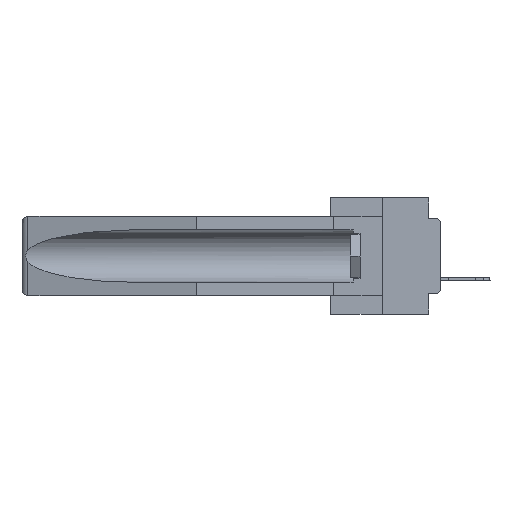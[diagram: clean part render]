
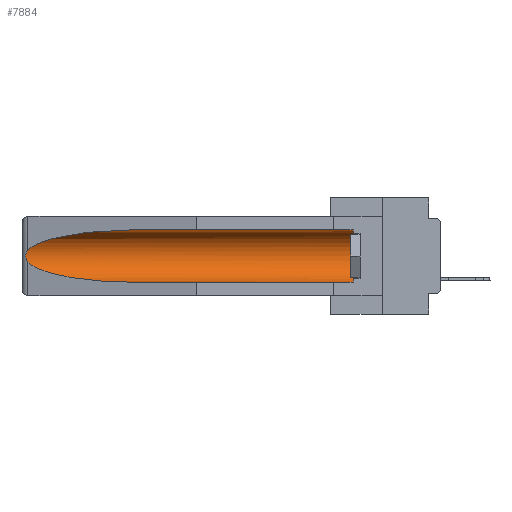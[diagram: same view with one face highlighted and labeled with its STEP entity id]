
A CAD part, left-side view. The second image highlights one B-rep face of the part: STEP entity #7884.
In plain terms, the highlighted cylindrical face has radius 2.857 mm (diameter 5.715 mm), a partial arc.
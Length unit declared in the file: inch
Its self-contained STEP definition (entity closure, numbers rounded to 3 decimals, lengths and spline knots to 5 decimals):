
#399 = CARTESIAN_POINT ( 'NONE',  ( 0.26537, 1.52718, -0.14972 ) ) ;
#456 = VECTOR ( 'NONE', #26872, 39.37008 ) ;
#866 = CARTESIAN_POINT ( 'NONE',  ( 0.155, -0.30754, -0.284 ) ) ;
#1058 = LINE ( 'NONE', #33928, #4656 ) ;
#1712 = VERTEX_POINT ( 'NONE', #8143 ) ;
#2428 = CARTESIAN_POINT ( 'NONE',  ( 0.155, 1.07973, -0.284 ) ) ;
#3092 = AXIS2_PLACEMENT_3D ( 'NONE', #14240, #19662, #25760 ) ;
#3195 = ORIENTED_EDGE ( 'NONE', *, *, #32228, .T. ) ;
#4011 = CARTESIAN_POINT ( 'NONE',  ( 0.25451, 1.48313, -0.09465 ) ) ;
#4656 = VECTOR ( 'NONE', #8696, 39.37008 ) ;
#5675 = CARTESIAN_POINT ( 'NONE',  ( 0.26537, 1.52718, -0.19328 ) ) ;
#5795 = CARTESIAN_POINT ( 'NONE',  ( 0.2673, 1.53269, -0.17917 ) ) ;
#6027 =( BOUNDED_CURVE ( )  B_SPLINE_CURVE ( 3, ( #21698, #19061, #21959, #36262 ),
 .UNSPECIFIED., .F., .F. ) 
 B_SPLINE_CURVE_WITH_KNOTS ( ( 4, 4 ),
 ( 0.1948, 1.5708 ),
 .UNSPECIFIED. ) 
 CURVE ( )  GEOMETRIC_REPRESENTATION_ITEM ( )  RATIONAL_B_SPLINE_CURVE ( ( 1., 0.848, 0.848, 1. ) ) 
 REPRESENTATION_ITEM ( '' )  );
#6773 = EDGE_CURVE ( 'NONE', #31456, #27522, #19392, .T. ) ;
#7884 = ADVANCED_FACE ( 'NONE', ( #23333 ), #31777, .F. ) ;
#8102 = DIRECTION ( 'NONE',  ( 0., -1., 0. ) ) ;
#8143 = CARTESIAN_POINT ( 'NONE',  ( 0.26537, 1.52718, -0.14972 ) ) ;
#8635 = CARTESIAN_POINT ( 'NONE',  ( 0.26597, 1.52961, -0.15275 ) ) ;
#8696 = DIRECTION ( 'NONE',  ( 0., 1., 0. ) ) ;
#9082 = EDGE_LOOP ( 'NONE', ( #19834, #3195, #24317, #28742, #28329, #35684 ) ) ;
#9541 = CARTESIAN_POINT ( 'NONE',  ( 0.155, 0.126, -0.059 ) ) ;
#9886 =( BOUNDED_CURVE ( )  B_SPLINE_CURVE ( 3, ( #35349, #21037, #4011, #18370 ),
 .UNSPECIFIED., .F., .F. ) 
 B_SPLINE_CURVE_WITH_KNOTS ( ( 4, 4 ),
 ( 4.71239, 6.08839 ),
 .UNSPECIFIED. ) 
 CURVE ( )  GEOMETRIC_REPRESENTATION_ITEM ( )  RATIONAL_B_SPLINE_CURVE ( ( 1., 0.848, 0.848, 1. ) ) 
 REPRESENTATION_ITEM ( '' )  );
#10415 = AXIS2_PLACEMENT_3D ( 'NONE', #17040, #8102, #32233 ) ;
#11491 = CARTESIAN_POINT ( 'NONE',  ( 0.2675, 1.53308, -0.16763 ) ) ;
#11739 = CARTESIAN_POINT ( 'NONE',  ( 0.2675, 1.53308, -0.17534 ) ) ;
#13542 = EDGE_CURVE ( 'NONE', #31456, #28046, #15192, .T. ) ;
#14240 = CARTESIAN_POINT ( 'NONE',  ( 0.155, -0.30754, -0.1715 ) ) ;
#14599 = CARTESIAN_POINT ( 'NONE',  ( 0.155, 1.07973, -0.059 ) ) ;
#15192 = LINE ( 'NONE', #866, #456 ) ;
#15440 = CARTESIAN_POINT ( 'NONE',  ( 0.26537, 1.52718, -0.19328 ) ) ;
#17040 = CARTESIAN_POINT ( 'NONE',  ( 0.155, 0.126, -0.1715 ) ) ;
#18370 = CARTESIAN_POINT ( 'NONE',  ( 0.26537, 1.52718, -0.14972 ) ) ;
#19061 = CARTESIAN_POINT ( 'NONE',  ( 0.25451, 1.48313, -0.24835 ) ) ;
#19392 = CIRCLE ( 'NONE', #10415, 0.1125 ) ;
#19662 = DIRECTION ( 'NONE',  ( 0., 1., 0. ) ) ;
#19834 = ORIENTED_EDGE ( 'NONE', *, *, #28846, .T. ) ;
#20890 = EDGE_CURVE ( 'NONE', #36007, #28046, #6027, .T. ) ;
#21037 = CARTESIAN_POINT ( 'NONE',  ( 0.21114, 1.30732, -0.059 ) ) ;
#21698 = CARTESIAN_POINT ( 'NONE',  ( 0.26537, 1.52718, -0.19328 ) ) ;
#21959 = CARTESIAN_POINT ( 'NONE',  ( 0.21114, 1.30732, -0.284 ) ) ;
#23231 = B_SPLINE_CURVE_WITH_KNOTS ( 'NONE', 3,
 ( #399, #8635, #34379, #34258, #11491, #11739, #5795, #23291, #26029, #5675 ),
 .UNSPECIFIED., .F., .F.,
 ( 4, 2, 2, 2, 4 ),
 ( 0., 0.00029, 0.00058, 0.00087, 0.00117 ),
 .UNSPECIFIED. ) ;
#23291 = CARTESIAN_POINT ( 'NONE',  ( 0.26655, 1.53094, -0.18657 ) ) ;
#23333 = FACE_OUTER_BOUND ( 'NONE', #9082, .T. ) ;
#23734 = VERTEX_POINT ( 'NONE', #14599 ) ;
#24317 = ORIENTED_EDGE ( 'NONE', *, *, #20890, .T. ) ;
#25760 = DIRECTION ( 'NONE',  ( 0., 0., 1. ) ) ;
#26029 = CARTESIAN_POINT ( 'NONE',  ( 0.26597, 1.5296, -0.19026 ) ) ;
#26872 = DIRECTION ( 'NONE',  ( 0., 1., 0. ) ) ;
#27522 = VERTEX_POINT ( 'NONE', #9541 ) ;
#28046 = VERTEX_POINT ( 'NONE', #2428 ) ;
#28329 = ORIENTED_EDGE ( 'NONE', *, *, #6773, .T. ) ;
#28742 = ORIENTED_EDGE ( 'NONE', *, *, #13542, .F. ) ;
#28846 = EDGE_CURVE ( 'NONE', #23734, #1712, #9886, .T. ) ;
#30386 = EDGE_CURVE ( 'NONE', #27522, #23734, #1058, .T. ) ;
#31456 = VERTEX_POINT ( 'NONE', #32303 ) ;
#31777 = CYLINDRICAL_SURFACE ( 'NONE', #3092, 0.1125 ) ;
#32228 = EDGE_CURVE ( 'NONE', #1712, #36007, #23231, .T. ) ;
#32233 = DIRECTION ( 'NONE',  ( 0., 0., 1. ) ) ;
#32303 = CARTESIAN_POINT ( 'NONE',  ( 0.155, 0.126, -0.284 ) ) ;
#33928 = CARTESIAN_POINT ( 'NONE',  ( 0.155, -0.30754, -0.059 ) ) ;
#34258 = CARTESIAN_POINT ( 'NONE',  ( 0.2673, 1.5327, -0.16383 ) ) ;
#34379 = CARTESIAN_POINT ( 'NONE',  ( 0.26654, 1.53092, -0.15636 ) ) ;
#35349 = CARTESIAN_POINT ( 'NONE',  ( 0.155, 1.07973, -0.059 ) ) ;
#35684 = ORIENTED_EDGE ( 'NONE', *, *, #30386, .T. ) ;
#36007 = VERTEX_POINT ( 'NONE', #15440 ) ;
#36262 = CARTESIAN_POINT ( 'NONE',  ( 0.155, 1.07973, -0.284 ) ) ;
